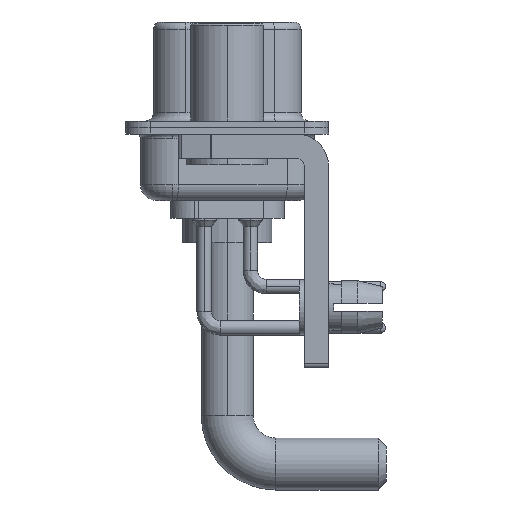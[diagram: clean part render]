
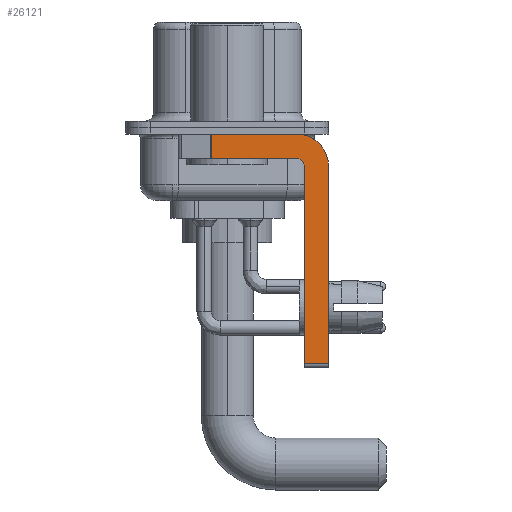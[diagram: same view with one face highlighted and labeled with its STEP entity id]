
A CAD part, left-side view. The second image highlights one B-rep face of the part: STEP entity #26121.
In plain terms, the highlighted planar face has unit normal (-1, 0, 0).
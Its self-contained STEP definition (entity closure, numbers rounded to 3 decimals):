
#224 = LINE ( 'NONE', #9287, #24087 ) ;
#560 = AXIS2_PLACEMENT_3D ( 'NONE', #27005, #22532, #27156 ) ;
#672 = ORIENTED_EDGE ( 'NONE', *, *, #28512, .F. ) ;
#722 = VECTOR ( 'NONE', #13369, 1000. ) ;
#904 = CARTESIAN_POINT ( 'NONE',  ( -2.9, -4.75, -2.4 ) ) ;
#916 = ORIENTED_EDGE ( 'NONE', *, *, #4738, .F. ) ;
#1866 = CARTESIAN_POINT ( 'NONE',  ( -2.9, -4.25, -2.4 ) ) ;
#1882 = EDGE_CURVE ( 'NONE', #17894, #25668, #6639, .T. ) ;
#2013 = PLANE ( 'NONE',  #21640 ) ;
#2456 = DIRECTION ( 'NONE',  ( 1., 0., 0. ) ) ;
#2812 = VERTEX_POINT ( 'NONE', #15698 ) ;
#3365 = ORIENTED_EDGE ( 'NONE', *, *, #21238, .F. ) ;
#4738 = EDGE_CURVE ( 'NONE', #10740, #13200, #16230, .T. ) ;
#4902 = VERTEX_POINT ( 'NONE', #17091 ) ;
#5190 = CARTESIAN_POINT ( 'NONE',  ( -2.9, -4.25, -1.9 ) ) ;
#5698 = ORIENTED_EDGE ( 'NONE', *, *, #7551, .F. ) ;
#6639 = LINE ( 'NONE', #11716, #722 ) ;
#6662 = VERTEX_POINT ( 'NONE', #23624 ) ;
#6753 = CARTESIAN_POINT ( 'NONE',  ( -2.9, 3., -0.4 ) ) ;
#7551 = EDGE_CURVE ( 'NONE', #6662, #25668, #19226, .T. ) ;
#7674 = CIRCLE ( 'NONE', #560, 0.5 ) ;
#8336 = CIRCLE ( 'NONE', #15958, 2. ) ;
#8497 = CARTESIAN_POINT ( 'NONE',  ( -2.9, -4.75, -14.8 ) ) ;
#9287 = CARTESIAN_POINT ( 'NONE',  ( -2.9, 0.978, -1.9 ) ) ;
#9292 = DIRECTION ( 'NONE',  ( 0., 0., -1. ) ) ;
#9753 = CARTESIAN_POINT ( 'NONE',  ( -2.9, -4.75, -14.55 ) ) ;
#10333 = EDGE_CURVE ( 'NONE', #2812, #13200, #224, .T. ) ;
#10740 = VERTEX_POINT ( 'NONE', #19676 ) ;
#10811 = EDGE_CURVE ( 'NONE', #17894, #10942, #24283, .T. ) ;
#10942 = VERTEX_POINT ( 'NONE', #904 ) ;
#11716 = CARTESIAN_POINT ( 'NONE',  ( -2.9, -4.25, -14.55 ) ) ;
#12242 = CARTESIAN_POINT ( 'NONE',  ( -2.9, -6.25, -2.4 ) ) ;
#12878 = DIRECTION ( 'NONE',  ( 1., 0., 0. ) ) ;
#13030 = FACE_OUTER_BOUND ( 'NONE', #24529, .T. ) ;
#13200 = VERTEX_POINT ( 'NONE', #18521 ) ;
#13369 = DIRECTION ( 'NONE',  ( 0., -1., 0. ) ) ;
#15277 = CARTESIAN_POINT ( 'NONE',  ( -2.9, -6.25, -14.55 ) ) ;
#15495 = VECTOR ( 'NONE', #15847, 1000. ) ;
#15698 = CARTESIAN_POINT ( 'NONE',  ( -2.9, 0.978, -0.4 ) ) ;
#15847 = DIRECTION ( 'NONE',  ( 0., -1., 0. ) ) ;
#15958 = AXIS2_PLACEMENT_3D ( 'NONE', #22846, #2456, #9292 ) ;
#16230 = LINE ( 'NONE', #5190, #20757 ) ;
#16854 = EDGE_CURVE ( 'NONE', #10942, #10740, #7674, .T. ) ;
#17091 = CARTESIAN_POINT ( 'NONE',  ( -2.9, -4.25, -0.4 ) ) ;
#17894 = VERTEX_POINT ( 'NONE', #9753 ) ;
#18521 = CARTESIAN_POINT ( 'NONE',  ( -2.9, 0.978, -1.9 ) ) ;
#18894 = VECTOR ( 'NONE', #28313, 1000. ) ;
#19226 = LINE ( 'NONE', #12242, #18894 ) ;
#19676 = CARTESIAN_POINT ( 'NONE',  ( -2.9, -4.25, -1.9 ) ) ;
#20019 = DIRECTION ( 'NONE',  ( 0., 0., -1. ) ) ;
#20757 = VECTOR ( 'NONE', #27404, 1000. ) ;
#21038 = DIRECTION ( 'NONE',  ( 0., 0., -1. ) ) ;
#21238 = EDGE_CURVE ( 'NONE', #4902, #6662, #8336, .T. ) ;
#21640 = AXIS2_PLACEMENT_3D ( 'NONE', #1866, #12878, #20019 ) ;
#22196 = DIRECTION ( 'NONE',  ( 0., 0., 1. ) ) ;
#22532 = DIRECTION ( 'NONE',  ( -1., 0., 0. ) ) ;
#22549 = LINE ( 'NONE', #6753, #15495 ) ;
#22846 = CARTESIAN_POINT ( 'NONE',  ( -2.9, -4.25, -2.4 ) ) ;
#23624 = CARTESIAN_POINT ( 'NONE',  ( -2.9, -6.25, -2.4 ) ) ;
#24087 = VECTOR ( 'NONE', #21038, 1000. ) ;
#24283 = LINE ( 'NONE', #8497, #24577 ) ;
#24345 = ORIENTED_EDGE ( 'NONE', *, *, #16854, .F. ) ;
#24529 = EDGE_LOOP ( 'NONE', ( #672, #26997, #916, #24345, #28947, #29270, #5698, #3365 ) ) ;
#24577 = VECTOR ( 'NONE', #22196, 1000. ) ;
#25668 = VERTEX_POINT ( 'NONE', #15277 ) ;
#26121 = ADVANCED_FACE ( 'NONE', ( #13030 ), #2013, .F. ) ;
#26997 = ORIENTED_EDGE ( 'NONE', *, *, #10333, .T. ) ;
#27005 = CARTESIAN_POINT ( 'NONE',  ( -2.9, -4.25, -2.4 ) ) ;
#27156 = DIRECTION ( 'NONE',  ( 0., 0., 1. ) ) ;
#27404 = DIRECTION ( 'NONE',  ( 0., 1., 0. ) ) ;
#28313 = DIRECTION ( 'NONE',  ( 0., 0., -1. ) ) ;
#28512 = EDGE_CURVE ( 'NONE', #2812, #4902, #22549, .T. ) ;
#28947 = ORIENTED_EDGE ( 'NONE', *, *, #10811, .F. ) ;
#29270 = ORIENTED_EDGE ( 'NONE', *, *, #1882, .T. ) ;
